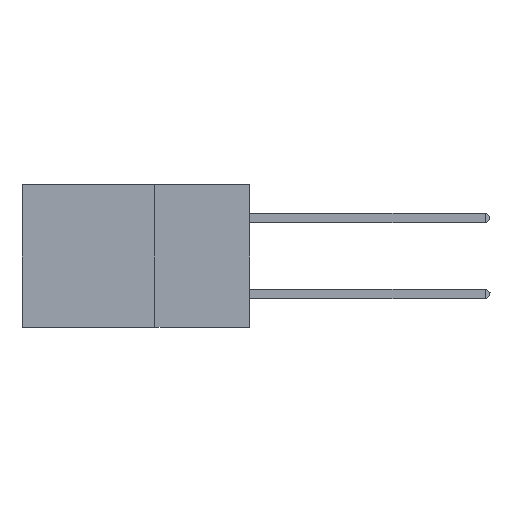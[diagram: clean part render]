
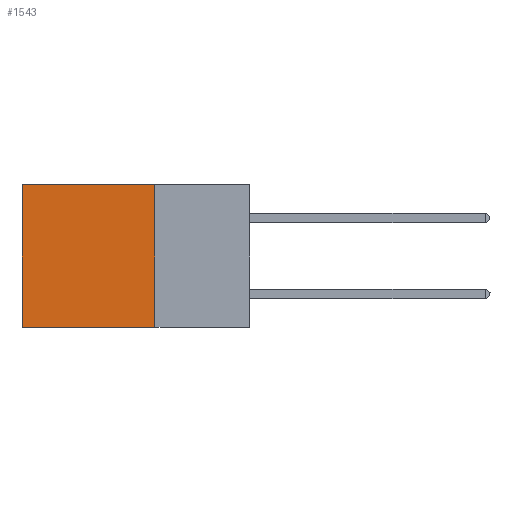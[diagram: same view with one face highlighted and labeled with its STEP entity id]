
A CAD part, left-side view. The second image highlights one B-rep face of the part: STEP entity #1543.
In plain terms, the highlighted planar face has unit normal (-1, 0, 0).
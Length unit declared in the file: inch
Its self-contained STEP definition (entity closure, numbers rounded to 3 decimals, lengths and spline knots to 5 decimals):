
#76 = DIRECTION ( 'NONE',  ( 0., 1., 0. ) ) ;
#231 = VECTOR ( 'NONE', #19968, 39.37008 ) ;
#1543 = ADVANCED_FACE ( 'NONE', ( #18132 ), #16159, .F. ) ;
#2128 = EDGE_CURVE ( 'NONE', #10887, #17904, #9693, .T. ) ;
#2783 = ORIENTED_EDGE ( 'NONE', *, *, #8768, .T. ) ;
#3027 = EDGE_LOOP ( 'NONE', ( #2783, #17801, #6982, #11458 ) ) ;
#4084 = CARTESIAN_POINT ( 'NONE',  ( 0.2875, 0.25, -0.375 ) ) ;
#4472 = DIRECTION ( 'NONE',  ( 1., 0., 0. ) ) ;
#4547 = CARTESIAN_POINT ( 'NONE',  ( 0.2875, 0.6, 0. ) ) ;
#6982 = ORIENTED_EDGE ( 'NONE', *, *, #2128, .F. ) ;
#7851 = EDGE_CURVE ( 'NONE', #10887, #9733, #15106, .T. ) ;
#8096 = LINE ( 'NONE', #20471, #12840 ) ;
#8105 = VECTOR ( 'NONE', #17625, 39.37008 ) ;
#8294 = CARTESIAN_POINT ( 'NONE',  ( 0.2875, 0.25, -0.375 ) ) ;
#8742 = DIRECTION ( 'NONE',  ( 0., 0., -1. ) ) ;
#8768 = EDGE_CURVE ( 'NONE', #9733, #13263, #8096, .T. ) ;
#9693 = LINE ( 'NONE', #4084, #8105 ) ;
#9733 = VERTEX_POINT ( 'NONE', #4547 ) ;
#10887 = VERTEX_POINT ( 'NONE', #14948 ) ;
#11458 = ORIENTED_EDGE ( 'NONE', *, *, #7851, .T. ) ;
#12636 = EDGE_CURVE ( 'NONE', #17904, #13263, #20105, .T. ) ;
#12840 = VECTOR ( 'NONE', #8742, 39.37008 ) ;
#12854 = AXIS2_PLACEMENT_3D ( 'NONE', #21324, #4472, #21252 ) ;
#13263 = VERTEX_POINT ( 'NONE', #15547 ) ;
#13410 = CARTESIAN_POINT ( 'NONE',  ( 0.2875, 0.25, 0. ) ) ;
#14504 = VECTOR ( 'NONE', #76, 39.37008 ) ;
#14948 = CARTESIAN_POINT ( 'NONE',  ( 0.2875, 0.25, 0. ) ) ;
#15106 = LINE ( 'NONE', #13410, #14504 ) ;
#15547 = CARTESIAN_POINT ( 'NONE',  ( 0.2875, 0.6, -0.375 ) ) ;
#16159 = PLANE ( 'NONE',  #12854 ) ;
#17625 = DIRECTION ( 'NONE',  ( 0., 0., -1. ) ) ;
#17801 = ORIENTED_EDGE ( 'NONE', *, *, #12636, .F. ) ;
#17904 = VERTEX_POINT ( 'NONE', #20444 ) ;
#18132 = FACE_OUTER_BOUND ( 'NONE', #3027, .T. ) ;
#19968 = DIRECTION ( 'NONE',  ( 0., 1., 0. ) ) ;
#20105 = LINE ( 'NONE', #8294, #231 ) ;
#20444 = CARTESIAN_POINT ( 'NONE',  ( 0.2875, 0.25, -0.375 ) ) ;
#20471 = CARTESIAN_POINT ( 'NONE',  ( 0.2875, 0.6, -0.375 ) ) ;
#21252 = DIRECTION ( 'NONE',  ( 0., 0., -1. ) ) ;
#21324 = CARTESIAN_POINT ( 'NONE',  ( 0.2875, 0.25, -0.375 ) ) ;
